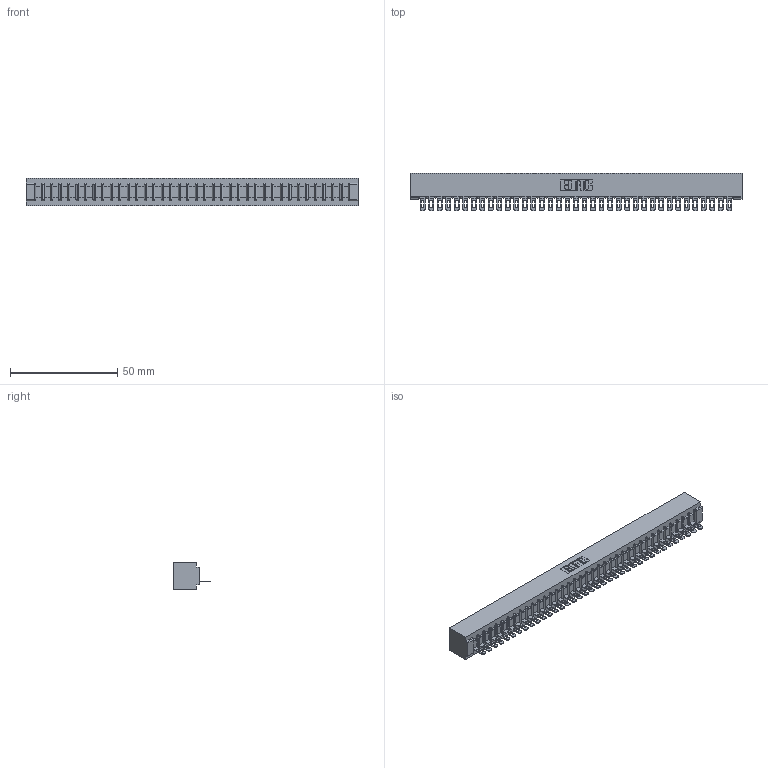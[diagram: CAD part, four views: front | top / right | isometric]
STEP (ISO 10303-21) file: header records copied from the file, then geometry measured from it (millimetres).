
FILE_DESCRIPTION (( 'STEP AP203' ), '1' );
FILE_NAME ('307-037-401-101.STEP', '2020-09-29T03:55:59', ( '' ), ( '' ), 'SwSTEP 2.0', 'SolidWorks 2020', '' );
FILE_SCHEMA (( 'CONFIG_CONTROL_DESIGN' ));
Length unit declared in the file: inch
Products named in the file (3): 307 Part_No Mounting Lugs; 307-037-401-101; 307-290-002_501
Assembly tree (38 placements, depth 2):
  307-037-401-101
    307 Part_No Mounting Lugs
    307-290-002_501  x37
Bounding box: 154.48 x 17.42 x 12.7 mm (x, y, z)
Volume: 17084.3 mm3; surface area: 21971.2 mm2
Topology: 38 solids, 38 shells, 2960 faces, 9105 edges, 5966 vertices
Faces by surface type: plane 1694, cylinder 1190, sphere 76
Entity records: 32852 total; most frequent: CARTESIAN_POINT 5540, ORIENTED_EDGE 5530, DIRECTION 5387, EDGE_CURVE 2765, LINE 2113, VECTOR 2113, VERTEX_POINT 1790, AXIS2_PLACEMENT_3D 1637
